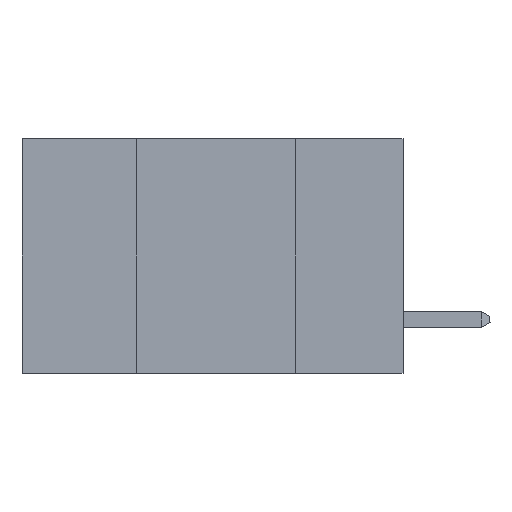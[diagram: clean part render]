
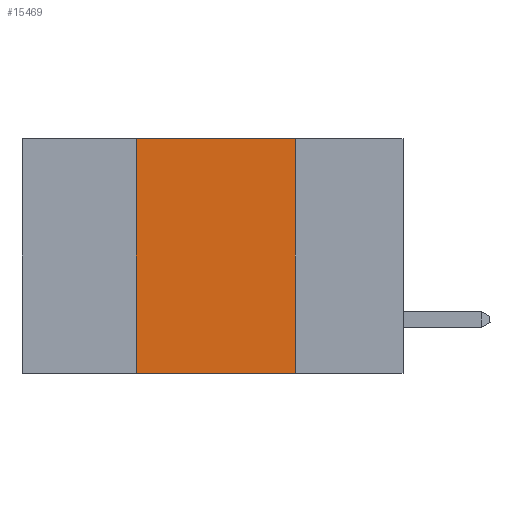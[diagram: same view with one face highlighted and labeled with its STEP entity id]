
A CAD part, left-side view. The second image highlights one B-rep face of the part: STEP entity #15469.
In plain terms, the highlighted planar face has unit normal (-1, 0, 0).
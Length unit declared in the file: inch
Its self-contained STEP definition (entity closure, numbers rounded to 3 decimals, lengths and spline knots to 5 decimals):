
#507 = CARTESIAN_POINT ( 'NONE',  ( 0., 0.17, -0.37 ) ) ;
#644 = LINE ( 'NONE', #30657, #10494 ) ;
#1477 = DIRECTION ( 'NONE',  ( 1., 0., 0. ) ) ;
#2529 = ORIENTED_EDGE ( 'NONE', *, *, #41586, .F. ) ;
#5708 = ORIENTED_EDGE ( 'NONE', *, *, #37211, .T. ) ;
#6280 = VECTOR ( 'NONE', #21304, 39.37008 ) ;
#6654 = LINE ( 'NONE', #13797, #31524 ) ;
#8147 = CARTESIAN_POINT ( 'NONE',  ( 0., 0.6, 0. ) ) ;
#8811 = EDGE_CURVE ( 'NONE', #31780, #19683, #644, .T. ) ;
#8889 = CARTESIAN_POINT ( 'NONE',  ( 0., 0.42, -0.37 ) ) ;
#9238 = CARTESIAN_POINT ( 'NONE',  ( 0., 0.42, 0. ) ) ;
#9403 = FACE_OUTER_BOUND ( 'NONE', #26125, .T. ) ;
#10494 = VECTOR ( 'NONE', #37724, 39.37008 ) ;
#10614 = VERTEX_POINT ( 'NONE', #507 ) ;
#11100 = AXIS2_PLACEMENT_3D ( 'NONE', #8147, #1477, #18408 ) ;
#12986 = LINE ( 'NONE', #21153, #6280 ) ;
#13797 = CARTESIAN_POINT ( 'NONE',  ( 0., 0.6, -0.37 ) ) ;
#13830 = ORIENTED_EDGE ( 'NONE', *, *, #25908, .F. ) ;
#14609 = CARTESIAN_POINT ( 'NONE',  ( 0., 0.17, 0. ) ) ;
#14674 = PLANE ( 'NONE',  #11100 ) ;
#15469 = ADVANCED_FACE ( 'NONE', ( #9403 ), #14674, .F. ) ;
#18408 = DIRECTION ( 'NONE',  ( 0., 0., -1. ) ) ;
#19292 = LINE ( 'NONE', #14609, #35822 ) ;
#19683 = VERTEX_POINT ( 'NONE', #27733 ) ;
#21153 = CARTESIAN_POINT ( 'NONE',  ( 0., 0.42, 0. ) ) ;
#21304 = DIRECTION ( 'NONE',  ( 0., 0., 1. ) ) ;
#25549 = DIRECTION ( 'NONE',  ( 0., 0., -1. ) ) ;
#25908 = EDGE_CURVE ( 'NONE', #19683, #10614, #19292, .T. ) ;
#26125 = EDGE_LOOP ( 'NONE', ( #13830, #27364, #2529, #5708 ) ) ;
#27364 = ORIENTED_EDGE ( 'NONE', *, *, #8811, .F. ) ;
#27733 = CARTESIAN_POINT ( 'NONE',  ( 0., 0.17, 0. ) ) ;
#30171 = DIRECTION ( 'NONE',  ( 0., -1., 0. ) ) ;
#30657 = CARTESIAN_POINT ( 'NONE',  ( 0., 0.6, 0. ) ) ;
#31524 = VECTOR ( 'NONE', #30171, 39.37008 ) ;
#31780 = VERTEX_POINT ( 'NONE', #9238 ) ;
#35822 = VECTOR ( 'NONE', #25549, 39.37008 ) ;
#37211 = EDGE_CURVE ( 'NONE', #37638, #10614, #6654, .T. ) ;
#37638 = VERTEX_POINT ( 'NONE', #8889 ) ;
#37724 = DIRECTION ( 'NONE',  ( 0., -1., 0. ) ) ;
#41586 = EDGE_CURVE ( 'NONE', #37638, #31780, #12986, .T. ) ;
